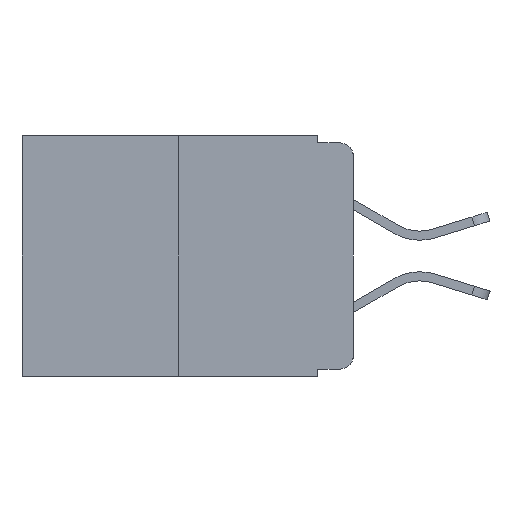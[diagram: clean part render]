
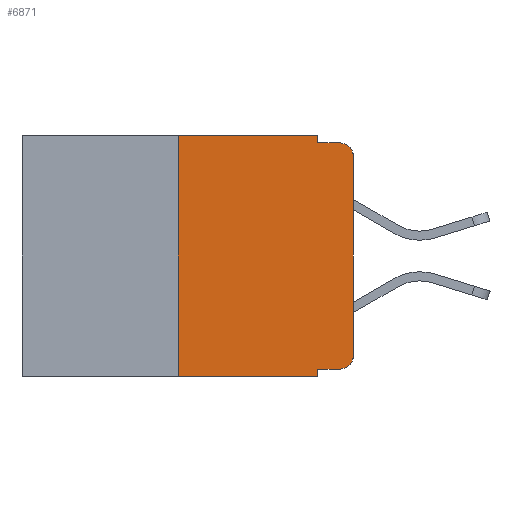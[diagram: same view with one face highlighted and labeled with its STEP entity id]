
A CAD part, left-side view. The second image highlights one B-rep face of the part: STEP entity #6871.
In plain terms, the highlighted planar face has unit normal (-1, 0, 0).
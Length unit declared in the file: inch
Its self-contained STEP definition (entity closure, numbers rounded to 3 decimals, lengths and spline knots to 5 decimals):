
#72 = DIRECTION ( 'NONE',  ( 0., 0., 1. ) ) ;
#500 = AXIS2_PLACEMENT_3D ( 'NONE', #8992, #14162, #2521 ) ;
#510 = PLANE ( 'NONE',  #15990 ) ;
#744 = CARTESIAN_POINT ( 'NONE',  ( 0., 0.051, -0.01 ) ) ;
#952 = CARTESIAN_POINT ( 'NONE',  ( 0., 0.051, -0.01 ) ) ;
#994 = CARTESIAN_POINT ( 'NONE',  ( 0., 0.051, -0.333 ) ) ;
#1099 = VECTOR ( 'NONE', #14637, 39.37008 ) ;
#1102 = DIRECTION ( 'NONE',  ( 0., 0., -1. ) ) ;
#1630 = DIRECTION ( 'NONE',  ( 0., -1., 0. ) ) ;
#2002 = CARTESIAN_POINT ( 'NONE',  ( 0., 0.051, -0.343 ) ) ;
#2190 = ORIENTED_EDGE ( 'NONE', *, *, #4546, .T. ) ;
#2521 = DIRECTION ( 'NONE',  ( 0., 0., -1. ) ) ;
#2769 = VECTOR ( 'NONE', #13182, 39.37008 ) ;
#2845 = LINE ( 'NONE', #13201, #1099 ) ;
#2983 = FACE_OUTER_BOUND ( 'NONE', #3451, .T. ) ;
#3079 = CARTESIAN_POINT ( 'NONE',  ( 0., 0., -0.313 ) ) ;
#3102 = VERTEX_POINT ( 'NONE', #2002 ) ;
#3275 = ORIENTED_EDGE ( 'NONE', *, *, #9961, .F. ) ;
#3409 = EDGE_CURVE ( 'NONE', #7370, #10034, #16169, .T. ) ;
#3418 = ORIENTED_EDGE ( 'NONE', *, *, #3409, .T. ) ;
#3451 = EDGE_LOOP ( 'NONE', ( #16714, #2190, #3275, #15497, #14380, #5363, #15279, #4259, #3418, #8029 ) ) ;
#4086 = EDGE_CURVE ( 'NONE', #8108, #11874, #14183, .T. ) ;
#4259 = ORIENTED_EDGE ( 'NONE', *, *, #7550, .F. ) ;
#4522 = LINE ( 'NONE', #5887, #16241 ) ;
#4546 = EDGE_CURVE ( 'NONE', #11874, #13424, #4576, .T. ) ;
#4550 = EDGE_CURVE ( 'NONE', #10888, #8107, #11438, .T. ) ;
#4576 = CIRCLE ( 'NONE', #500, 0.02 ) ;
#4586 = DIRECTION ( 'NONE',  ( 1., 0., 0. ) ) ;
#4997 = CARTESIAN_POINT ( 'NONE',  ( 0., 0.051, 0. ) ) ;
#5057 = VECTOR ( 'NONE', #13057, 39.37008 ) ;
#5363 = ORIENTED_EDGE ( 'NONE', *, *, #4550, .F. ) ;
#5460 = CARTESIAN_POINT ( 'NONE',  ( 0., 0.25, 0. ) ) ;
#5461 = CARTESIAN_POINT ( 'NONE',  ( 0., 0.473, 0. ) ) ;
#5887 = CARTESIAN_POINT ( 'NONE',  ( 0., 0.473, -0.343 ) ) ;
#5903 = DIRECTION ( 'NONE',  ( 0., -1., 0. ) ) ;
#5992 = CIRCLE ( 'NONE', #13317, 0.02 ) ;
#6591 = EDGE_CURVE ( 'NONE', #10888, #3102, #4522, .T. ) ;
#6871 = ADVANCED_FACE ( 'NONE', ( #2983 ), #510, .F. ) ;
#6913 = CARTESIAN_POINT ( 'NONE',  ( 0., 0.02, -0.01 ) ) ;
#7139 = VERTEX_POINT ( 'NONE', #9103 ) ;
#7370 = VERTEX_POINT ( 'NONE', #994 ) ;
#7550 = EDGE_CURVE ( 'NONE', #7370, #3102, #14170, .T. ) ;
#8029 = ORIENTED_EDGE ( 'NONE', *, *, #13667, .T. ) ;
#8107 = VERTEX_POINT ( 'NONE', #5460 ) ;
#8108 = VERTEX_POINT ( 'NONE', #3079 ) ;
#8992 = CARTESIAN_POINT ( 'NONE',  ( 0., 0.02, -0.03 ) ) ;
#9103 = CARTESIAN_POINT ( 'NONE',  ( 0., 0.051, 0. ) ) ;
#9715 = CARTESIAN_POINT ( 'NONE',  ( 0., 0.25, -0.343 ) ) ;
#9961 = EDGE_CURVE ( 'NONE', #15523, #13424, #11821, .T. ) ;
#10034 = VERTEX_POINT ( 'NONE', #11370 ) ;
#10805 = LINE ( 'NONE', #5461, #2769 ) ;
#10888 = VERTEX_POINT ( 'NONE', #9715 ) ;
#11054 = DIRECTION ( 'NONE',  ( 0., -1., 0. ) ) ;
#11370 = CARTESIAN_POINT ( 'NONE',  ( 0., 0.02, -0.333 ) ) ;
#11438 = LINE ( 'NONE', #16625, #15701 ) ;
#11622 = VECTOR ( 'NONE', #72, 39.37008 ) ;
#11821 = LINE ( 'NONE', #744, #15489 ) ;
#11874 = VERTEX_POINT ( 'NONE', #13694 ) ;
#12274 = CARTESIAN_POINT ( 'NONE',  ( 0., 0.051, -0.333 ) ) ;
#12995 = EDGE_CURVE ( 'NONE', #7139, #15523, #2845, .T. ) ;
#13057 = DIRECTION ( 'NONE',  ( 0., 0., -1. ) ) ;
#13182 = DIRECTION ( 'NONE',  ( 0., -1., 0. ) ) ;
#13201 = CARTESIAN_POINT ( 'NONE',  ( 0., 0.051, 0. ) ) ;
#13317 = AXIS2_PLACEMENT_3D ( 'NONE', #14265, #16652, #1102 ) ;
#13424 = VERTEX_POINT ( 'NONE', #6913 ) ;
#13505 = CARTESIAN_POINT ( 'NONE',  ( 0., 0.473, 0. ) ) ;
#13667 = EDGE_CURVE ( 'NONE', #10034, #8108, #5992, .T. ) ;
#13694 = CARTESIAN_POINT ( 'NONE',  ( 0., 0., -0.03 ) ) ;
#14087 = CARTESIAN_POINT ( 'NONE',  ( 0., 0., 0. ) ) ;
#14162 = DIRECTION ( 'NONE',  ( -1., 0., 0. ) ) ;
#14170 = LINE ( 'NONE', #4997, #5057 ) ;
#14183 = LINE ( 'NONE', #14087, #11622 ) ;
#14244 = VECTOR ( 'NONE', #5903, 39.37008 ) ;
#14265 = CARTESIAN_POINT ( 'NONE',  ( 0., 0.02, -0.313 ) ) ;
#14380 = ORIENTED_EDGE ( 'NONE', *, *, #14621, .F. ) ;
#14610 = DIRECTION ( 'NONE',  ( 0., 0., -1. ) ) ;
#14621 = EDGE_CURVE ( 'NONE', #8107, #7139, #10805, .T. ) ;
#14637 = DIRECTION ( 'NONE',  ( 0., 0., -1. ) ) ;
#15279 = ORIENTED_EDGE ( 'NONE', *, *, #6591, .T. ) ;
#15343 = DIRECTION ( 'NONE',  ( 0., 0., 1. ) ) ;
#15489 = VECTOR ( 'NONE', #1630, 39.37008 ) ;
#15497 = ORIENTED_EDGE ( 'NONE', *, *, #12995, .F. ) ;
#15523 = VERTEX_POINT ( 'NONE', #952 ) ;
#15701 = VECTOR ( 'NONE', #15343, 39.37008 ) ;
#15990 = AXIS2_PLACEMENT_3D ( 'NONE', #13505, #4586, #14610 ) ;
#16169 = LINE ( 'NONE', #12274, #14244 ) ;
#16241 = VECTOR ( 'NONE', #11054, 39.37008 ) ;
#16625 = CARTESIAN_POINT ( 'NONE',  ( 0., 0.25, 0. ) ) ;
#16652 = DIRECTION ( 'NONE',  ( -1., 0., 0. ) ) ;
#16714 = ORIENTED_EDGE ( 'NONE', *, *, #4086, .T. ) ;
